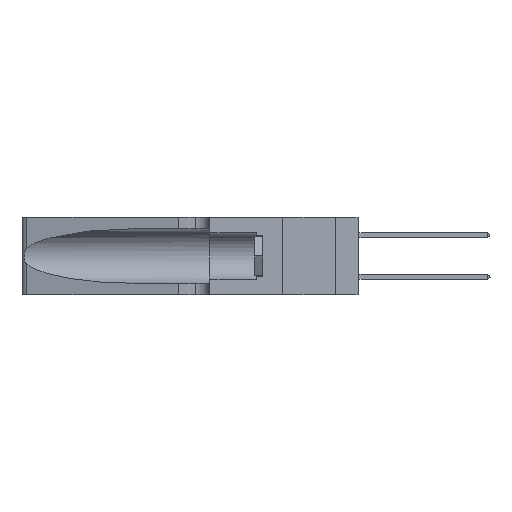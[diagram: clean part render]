
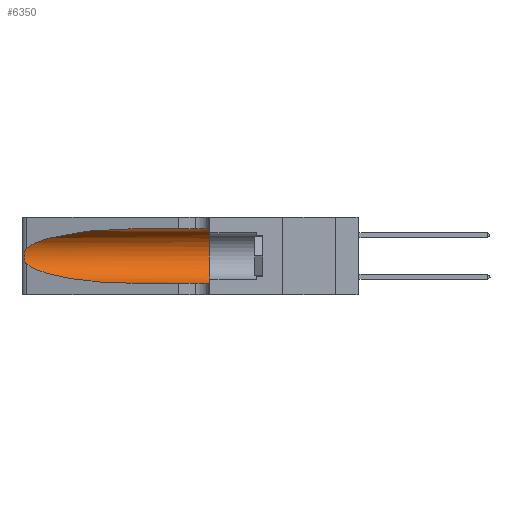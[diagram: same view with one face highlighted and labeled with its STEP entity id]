
A CAD part, left-side view. The second image highlights one B-rep face of the part: STEP entity #6350.
In plain terms, the highlighted cylindrical face has radius 3.308 mm (diameter 6.617 mm), a partial arc.
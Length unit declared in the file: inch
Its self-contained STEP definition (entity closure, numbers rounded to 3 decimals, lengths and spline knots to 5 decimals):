
#3127 = B_SPLINE_CURVE_WITH_KNOTS ( 'NONE', 3,
 ( #16273, #36157, #26398, #33108, #39966, #36978, #7588, #33788, #4598, #21196, #19879, #24629, #13439, #14108 ),
 .UNSPECIFIED., .F., .F.,
 ( 4, 2, 2, 2, 2, 2, 4 ),
 ( 0., 0.00027, 0.00053, 0.00107, 0.0016, 0.00187, 0.00214 ),
 .UNSPECIFIED. ) ;
#3850 = CARTESIAN_POINT ( 'NONE',  ( 0.1305, 1.61858, 0.185 ) ) ;
#3942 = DIRECTION ( 'NONE',  ( 0., -1., 0. ) ) ;
#4598 = CARTESIAN_POINT ( 'NONE',  ( 0.26017, 1.23833, 0.17102 ) ) ;
#4986 = CARTESIAN_POINT ( 'NONE',  ( 0.18966, 0.96281, 0.05475 ) ) ;
#5297 = ORIENTED_EDGE ( 'NONE', *, *, #28262, .T. ) ;
#5489 = CARTESIAN_POINT ( 'NONE',  ( 0.1305, 0.35, 0.05475 ) ) ;
#5789 = CARTESIAN_POINT ( 'NONE',  ( 0.1305, 0.35, 0.185 ) ) ;
#6214 = CARTESIAN_POINT ( 'NONE',  ( 0.1305, 0.72297, 0.31525 ) ) ;
#6350 = ADVANCED_FACE ( 'NONE', ( #38182 ), #6366, .F. ) ;
#6366 = CYLINDRICAL_SURFACE ( 'NONE', #28729, 0.13025 ) ;
#6377 = EDGE_LOOP ( 'NONE', ( #5297, #30839, #29923, #11442, #7812, #17622 ) ) ;
#6599 = VERTEX_POINT ( 'NONE', #24181 ) ;
#7588 = CARTESIAN_POINT ( 'NONE',  ( 0.26075, 1.23896, 0.19203 ) ) ;
#7812 = ORIENTED_EDGE ( 'NONE', *, *, #12652, .F. ) ;
#7961 = CARTESIAN_POINT ( 'NONE',  ( 0.25487, 1.22718, 0.14631 ) ) ;
#8806 = VECTOR ( 'NONE', #13997, 39.37008 ) ;
#9121 = CARTESIAN_POINT ( 'NONE',  ( 0.1305, 1.61858, 0.05475 ) ) ;
#9489 =( BOUNDED_CURVE ( )  B_SPLINE_CURVE ( 3, ( #7961, #11436, #4986, #24737 ),
 .UNSPECIFIED., .F., .T. ) 
 B_SPLINE_CURVE_WITH_KNOTS ( ( 4, 4 ),
 ( 3.44316, 4.71239 ),
 .UNSPECIFIED. ) 
 CURVE ( )  GEOMETRIC_REPRESENTATION_ITEM ( )  RATIONAL_B_SPLINE_CURVE ( ( 1., 0.87, 0.87, 1. ) ) 
 REPRESENTATION_ITEM ( '' )  );
#11436 = CARTESIAN_POINT ( 'NONE',  ( 0.2373, 1.15595, 0.08982 ) ) ;
#11442 = ORIENTED_EDGE ( 'NONE', *, *, #24428, .T. ) ;
#11564 = EDGE_CURVE ( 'NONE', #30177, #18064, #17465, .T. ) ;
#11996 = DIRECTION ( 'NONE',  ( 0., 1., 0. ) ) ;
#12080 = EDGE_CURVE ( 'NONE', #35882, #32891, #9489, .T. ) ;
#12652 = EDGE_CURVE ( 'NONE', #18064, #13425, #26149, .T. ) ;
#13425 = VERTEX_POINT ( 'NONE', #5489 ) ;
#13439 = CARTESIAN_POINT ( 'NONE',  ( 0.25555, 1.22993, 0.14849 ) ) ;
#13908 =( BOUNDED_CURVE ( )  B_SPLINE_CURVE ( 3, ( #16711, #34895, #29502, #40510 ),
 .UNSPECIFIED., .F., .F. ) 
 B_SPLINE_CURVE_WITH_KNOTS ( ( 4, 4 ),
 ( 1.5708, 2.84003 ),
 .UNSPECIFIED. ) 
 CURVE ( )  GEOMETRIC_REPRESENTATION_ITEM ( )  RATIONAL_B_SPLINE_CURVE ( ( 1., 0.87, 0.87, 1. ) ) 
 REPRESENTATION_ITEM ( '' )  );
#13997 = DIRECTION ( 'NONE',  ( 0., -1., 0. ) ) ;
#14108 = CARTESIAN_POINT ( 'NONE',  ( 0.25487, 1.22718, 0.14631 ) ) ;
#14255 = LINE ( 'NONE', #9121, #39381 ) ;
#15836 = CARTESIAN_POINT ( 'NONE',  ( 0.1305, 0.72297, 0.05475 ) ) ;
#16273 = CARTESIAN_POINT ( 'NONE',  ( 0.25487, 1.22718, 0.22369 ) ) ;
#16711 = CARTESIAN_POINT ( 'NONE',  ( 0.1305, 0.72297, 0.31525 ) ) ;
#17465 = LINE ( 'NONE', #23998, #8806 ) ;
#17622 = ORIENTED_EDGE ( 'NONE', *, *, #11564, .F. ) ;
#18064 = VERTEX_POINT ( 'NONE', #40769 ) ;
#19879 = CARTESIAN_POINT ( 'NONE',  ( 0.25789, 1.23486, 0.15765 ) ) ;
#20884 = DIRECTION ( 'NONE',  ( 0., 0., -1. ) ) ;
#21196 = CARTESIAN_POINT ( 'NONE',  ( 0.25856, 1.23593, 0.16098 ) ) ;
#23998 = CARTESIAN_POINT ( 'NONE',  ( 0.1305, 1.61858, 0.31525 ) ) ;
#24152 = AXIS2_PLACEMENT_3D ( 'NONE', #5789, #11996, #34871 ) ;
#24181 = CARTESIAN_POINT ( 'NONE',  ( 0.25487, 1.22718, 0.22369 ) ) ;
#24428 = EDGE_CURVE ( 'NONE', #32891, #13425, #14255, .T. ) ;
#24629 = CARTESIAN_POINT ( 'NONE',  ( 0.25639, 1.23186, 0.15144 ) ) ;
#24737 = CARTESIAN_POINT ( 'NONE',  ( 0.1305, 0.72297, 0.05475 ) ) ;
#24831 = DIRECTION ( 'NONE',  ( 0., -1., 0. ) ) ;
#26146 = EDGE_CURVE ( 'NONE', #6599, #35882, #3127, .T. ) ;
#26149 = CIRCLE ( 'NONE', #24152, 0.13025 ) ;
#26398 = CARTESIAN_POINT ( 'NONE',  ( 0.25639, 1.23184, 0.21858 ) ) ;
#28262 = EDGE_CURVE ( 'NONE', #30177, #6599, #13908, .T. ) ;
#28729 = AXIS2_PLACEMENT_3D ( 'NONE', #3850, #3942, #20884 ) ;
#29502 = CARTESIAN_POINT ( 'NONE',  ( 0.2373, 1.15595, 0.28018 ) ) ;
#29923 = ORIENTED_EDGE ( 'NONE', *, *, #12080, .T. ) ;
#29957 = CARTESIAN_POINT ( 'NONE',  ( 0.25487, 1.22718, 0.14631 ) ) ;
#30177 = VERTEX_POINT ( 'NONE', #6214 ) ;
#30839 = ORIENTED_EDGE ( 'NONE', *, *, #26146, .T. ) ;
#32891 = VERTEX_POINT ( 'NONE', #15836 ) ;
#33108 = CARTESIAN_POINT ( 'NONE',  ( 0.25787, 1.23484, 0.2124 ) ) ;
#33788 = CARTESIAN_POINT ( 'NONE',  ( 0.26075, 1.23896, 0.178 ) ) ;
#34871 = DIRECTION ( 'NONE',  ( 0., 0., 1. ) ) ;
#34895 = CARTESIAN_POINT ( 'NONE',  ( 0.18966, 0.96281, 0.31525 ) ) ;
#35882 = VERTEX_POINT ( 'NONE', #29957 ) ;
#36157 = CARTESIAN_POINT ( 'NONE',  ( 0.25555, 1.22994, 0.2215 ) ) ;
#36978 = CARTESIAN_POINT ( 'NONE',  ( 0.26018, 1.23835, 0.19895 ) ) ;
#38182 = FACE_OUTER_BOUND ( 'NONE', #6377, .T. ) ;
#39381 = VECTOR ( 'NONE', #24831, 39.37008 ) ;
#39966 = CARTESIAN_POINT ( 'NONE',  ( 0.25854, 1.2359, 0.20912 ) ) ;
#40510 = CARTESIAN_POINT ( 'NONE',  ( 0.25487, 1.22718, 0.22369 ) ) ;
#40769 = CARTESIAN_POINT ( 'NONE',  ( 0.1305, 0.35, 0.31525 ) ) ;
